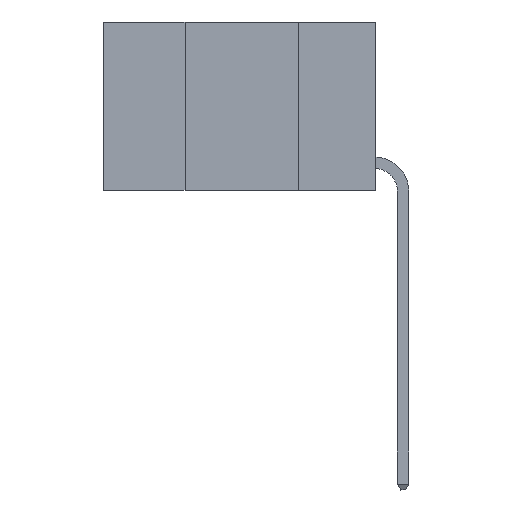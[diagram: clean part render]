
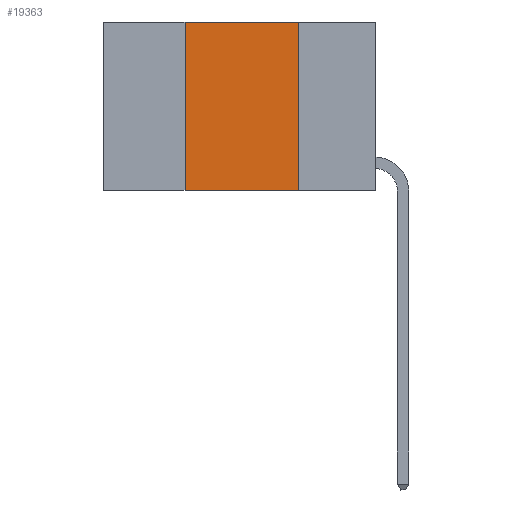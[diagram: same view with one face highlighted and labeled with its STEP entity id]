
A CAD part, left-side view. The second image highlights one B-rep face of the part: STEP entity #19363.
In plain terms, the highlighted planar face has unit normal (-1, 0, 0).
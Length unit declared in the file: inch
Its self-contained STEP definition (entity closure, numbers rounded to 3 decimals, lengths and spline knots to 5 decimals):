
#316 = VERTEX_POINT ( 'NONE', #5647 ) ;
#621 = CARTESIAN_POINT ( 'NONE',  ( 0., 0.17, 0. ) ) ;
#894 = CARTESIAN_POINT ( 'NONE',  ( 0., 0.6, 0. ) ) ;
#1044 = LINE ( 'NONE', #12172, #2259 ) ;
#2259 = VECTOR ( 'NONE', #23714, 39.37008 ) ;
#2291 = ORIENTED_EDGE ( 'NONE', *, *, #22480, .F. ) ;
#3261 = ORIENTED_EDGE ( 'NONE', *, *, #28547, .F. ) ;
#3670 = CARTESIAN_POINT ( 'NONE',  ( 0., 0.42, -0.37 ) ) ;
#5618 = DIRECTION ( 'NONE',  ( 0., 0., -1. ) ) ;
#5647 = CARTESIAN_POINT ( 'NONE',  ( 0., 0.17, -0.37 ) ) ;
#8042 = LINE ( 'NONE', #16724, #22893 ) ;
#8329 = VERTEX_POINT ( 'NONE', #621 ) ;
#9921 = EDGE_CURVE ( 'NONE', #8329, #316, #25689, .T. ) ;
#10572 = VECTOR ( 'NONE', #5618, 39.37008 ) ;
#12172 = CARTESIAN_POINT ( 'NONE',  ( 0., 0.6, -0.37 ) ) ;
#12290 = LINE ( 'NONE', #21208, #18880 ) ;
#12446 = DIRECTION ( 'NONE',  ( 1., 0., 0. ) ) ;
#12503 = EDGE_CURVE ( 'NONE', #24952, #316, #1044, .T. ) ;
#12752 = DIRECTION ( 'NONE',  ( 0., -1., 0. ) ) ;
#14510 = FACE_OUTER_BOUND ( 'NONE', #18305, .T. ) ;
#15596 = AXIS2_PLACEMENT_3D ( 'NONE', #894, #12446, #23279 ) ;
#16724 = CARTESIAN_POINT ( 'NONE',  ( 0., 0.6, 0. ) ) ;
#18305 = EDGE_LOOP ( 'NONE', ( #27448, #2291, #3261, #23611 ) ) ;
#18880 = VECTOR ( 'NONE', #19022, 39.37008 ) ;
#19022 = DIRECTION ( 'NONE',  ( 0., 0., 1. ) ) ;
#19363 = ADVANCED_FACE ( 'NONE', ( #14510 ), #25631, .F. ) ;
#20897 = VERTEX_POINT ( 'NONE', #22537 ) ;
#21208 = CARTESIAN_POINT ( 'NONE',  ( 0., 0.42, 0. ) ) ;
#22480 = EDGE_CURVE ( 'NONE', #20897, #8329, #8042, .T. ) ;
#22537 = CARTESIAN_POINT ( 'NONE',  ( 0., 0.42, 0. ) ) ;
#22893 = VECTOR ( 'NONE', #12752, 39.37008 ) ;
#23279 = DIRECTION ( 'NONE',  ( 0., 0., -1. ) ) ;
#23611 = ORIENTED_EDGE ( 'NONE', *, *, #12503, .T. ) ;
#23714 = DIRECTION ( 'NONE',  ( 0., -1., 0. ) ) ;
#23772 = CARTESIAN_POINT ( 'NONE',  ( 0., 0.17, 0. ) ) ;
#24952 = VERTEX_POINT ( 'NONE', #3670 ) ;
#25631 = PLANE ( 'NONE',  #15596 ) ;
#25689 = LINE ( 'NONE', #23772, #10572 ) ;
#27448 = ORIENTED_EDGE ( 'NONE', *, *, #9921, .F. ) ;
#28547 = EDGE_CURVE ( 'NONE', #24952, #20897, #12290, .T. ) ;
